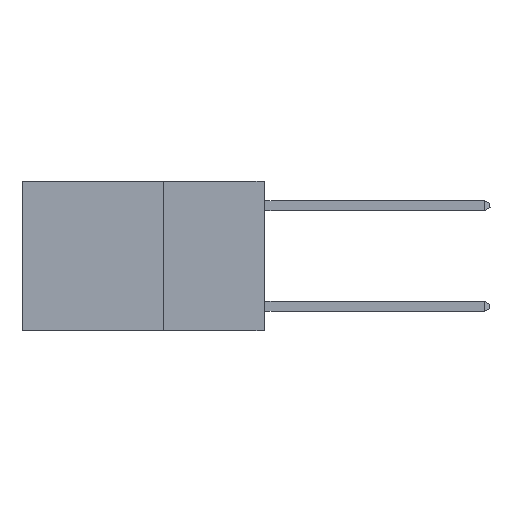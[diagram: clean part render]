
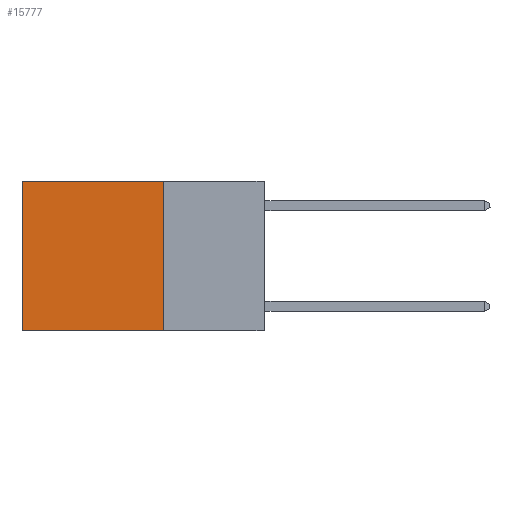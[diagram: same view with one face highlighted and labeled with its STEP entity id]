
A CAD part, left-side view. The second image highlights one B-rep face of the part: STEP entity #15777.
In plain terms, the highlighted planar face has unit normal (-1, 0, 0).
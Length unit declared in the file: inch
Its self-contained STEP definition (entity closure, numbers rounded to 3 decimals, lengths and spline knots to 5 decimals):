
#1058 = LINE ( 'NONE', #10189, #5413 ) ;
#1438 = VECTOR ( 'NONE', #15896, 39.37008 ) ;
#1784 = EDGE_LOOP ( 'NONE', ( #9576, #8662, #14092, #15363 ) ) ;
#2095 = DIRECTION ( 'NONE',  ( 0., 0., -1. ) ) ;
#2764 = CARTESIAN_POINT ( 'NONE',  ( 0.2625, 0.6, -0.37 ) ) ;
#3276 = CARTESIAN_POINT ( 'NONE',  ( 0.2625, 0.25, -0.37 ) ) ;
#3316 = VERTEX_POINT ( 'NONE', #3528 ) ;
#3500 = EDGE_CURVE ( 'NONE', #6679, #15564, #11933, .T. ) ;
#3528 = CARTESIAN_POINT ( 'NONE',  ( 0.2625, 0.25, 0. ) ) ;
#3708 = DIRECTION ( 'NONE',  ( 0., 1., 0. ) ) ;
#5214 = LINE ( 'NONE', #6249, #11461 ) ;
#5376 = CARTESIAN_POINT ( 'NONE',  ( 0.2625, 0.25, -0.37 ) ) ;
#5413 = VECTOR ( 'NONE', #3708, 39.37008 ) ;
#5582 = DIRECTION ( 'NONE',  ( 1., 0., 0. ) ) ;
#6249 = CARTESIAN_POINT ( 'NONE',  ( 0.2625, 0.25, 0. ) ) ;
#6679 = VERTEX_POINT ( 'NONE', #3276 ) ;
#6879 = PLANE ( 'NONE',  #14241 ) ;
#7560 = VECTOR ( 'NONE', #2095, 39.37008 ) ;
#8586 = VERTEX_POINT ( 'NONE', #12815 ) ;
#8662 = ORIENTED_EDGE ( 'NONE', *, *, #3500, .F. ) ;
#9576 = ORIENTED_EDGE ( 'NONE', *, *, #12673, .T. ) ;
#10189 = CARTESIAN_POINT ( 'NONE',  ( 0.2625, 0.25, 0. ) ) ;
#10498 = DIRECTION ( 'NONE',  ( 0., 0., -1. ) ) ;
#10847 = DIRECTION ( 'NONE',  ( 0., 0., -1. ) ) ;
#11301 = LINE ( 'NONE', #16450, #7560 ) ;
#11461 = VECTOR ( 'NONE', #10498, 39.37008 ) ;
#11933 = LINE ( 'NONE', #5376, #1438 ) ;
#12141 = CARTESIAN_POINT ( 'NONE',  ( 0.2625, 0.25, 0. ) ) ;
#12673 = EDGE_CURVE ( 'NONE', #8586, #15564, #11301, .T. ) ;
#12815 = CARTESIAN_POINT ( 'NONE',  ( 0.2625, 0.6, 0. ) ) ;
#13428 = FACE_OUTER_BOUND ( 'NONE', #1784, .T. ) ;
#14092 = ORIENTED_EDGE ( 'NONE', *, *, #14862, .F. ) ;
#14241 = AXIS2_PLACEMENT_3D ( 'NONE', #12141, #5582, #10847 ) ;
#14862 = EDGE_CURVE ( 'NONE', #3316, #6679, #5214, .T. ) ;
#15363 = ORIENTED_EDGE ( 'NONE', *, *, #15433, .T. ) ;
#15433 = EDGE_CURVE ( 'NONE', #3316, #8586, #1058, .T. ) ;
#15564 = VERTEX_POINT ( 'NONE', #2764 ) ;
#15777 = ADVANCED_FACE ( 'NONE', ( #13428 ), #6879, .F. ) ;
#15896 = DIRECTION ( 'NONE',  ( 0., 1., 0. ) ) ;
#16450 = CARTESIAN_POINT ( 'NONE',  ( 0.2625, 0.6, 0. ) ) ;
